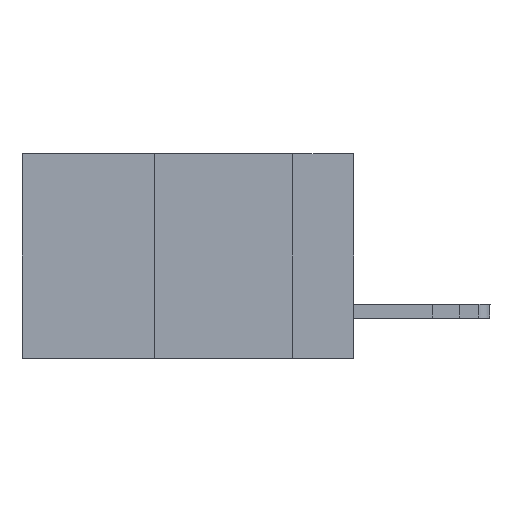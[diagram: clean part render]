
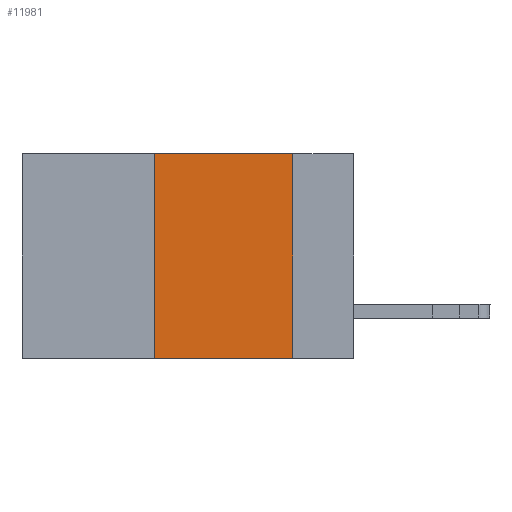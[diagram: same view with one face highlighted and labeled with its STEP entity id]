
A CAD part, left-side view. The second image highlights one B-rep face of the part: STEP entity #11981.
In plain terms, the highlighted planar face has unit normal (-1, 0, 0).
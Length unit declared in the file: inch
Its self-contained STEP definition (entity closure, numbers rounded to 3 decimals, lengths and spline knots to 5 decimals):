
#459 = ORIENTED_EDGE ( 'NONE', *, *, #1982, .F. ) ;
#484 = ORIENTED_EDGE ( 'NONE', *, *, #7917, .F. ) ;
#525 = CARTESIAN_POINT ( 'NONE',  ( 0., 0.6, 0. ) ) ;
#664 = ORIENTED_EDGE ( 'NONE', *, *, #16163, .T. ) ;
#945 = CARTESIAN_POINT ( 'NONE',  ( 0., 0.36, 0. ) ) ;
#1166 = CARTESIAN_POINT ( 'NONE',  ( 0., 0.11, 0. ) ) ;
#1393 = VERTEX_POINT ( 'NONE', #12732 ) ;
#1544 = EDGE_LOOP ( 'NONE', ( #459, #9852, #484, #664 ) ) ;
#1982 = EDGE_CURVE ( 'NONE', #1393, #10221, #14683, .T. ) ;
#2704 = VERTEX_POINT ( 'NONE', #945 ) ;
#2792 = PLANE ( 'NONE',  #5031 ) ;
#3411 = CARTESIAN_POINT ( 'NONE',  ( 0., 0.6, -0.37 ) ) ;
#4093 = DIRECTION ( 'NONE',  ( 0., 0., -1. ) ) ;
#4200 = DIRECTION ( 'NONE',  ( 1., 0., 0. ) ) ;
#4222 = DIRECTION ( 'NONE',  ( 0., -1., 0. ) ) ;
#5031 = AXIS2_PLACEMENT_3D ( 'NONE', #11901, #4200, #4093 ) ;
#5520 = CARTESIAN_POINT ( 'NONE',  ( 0., 0.11, -0.37 ) ) ;
#6100 = VECTOR ( 'NONE', #12401, 39.37008 ) ;
#6307 = DIRECTION ( 'NONE',  ( 0., 0., -1. ) ) ;
#7917 = EDGE_CURVE ( 'NONE', #14417, #2704, #11323, .T. ) ;
#9029 = VECTOR ( 'NONE', #6307, 39.37008 ) ;
#9341 = DIRECTION ( 'NONE',  ( 0., 0., 1. ) ) ;
#9852 = ORIENTED_EDGE ( 'NONE', *, *, #11489, .F. ) ;
#10125 = CARTESIAN_POINT ( 'NONE',  ( 0., 0.36, -0.37 ) ) ;
#10221 = VERTEX_POINT ( 'NONE', #5520 ) ;
#10917 = VECTOR ( 'NONE', #4222, 39.37008 ) ;
#11323 = LINE ( 'NONE', #15772, #14731 ) ;
#11489 = EDGE_CURVE ( 'NONE', #2704, #1393, #14545, .T. ) ;
#11901 = CARTESIAN_POINT ( 'NONE',  ( 0., 0.6, 0. ) ) ;
#11981 = ADVANCED_FACE ( 'NONE', ( #13102 ), #2792, .F. ) ;
#12401 = DIRECTION ( 'NONE',  ( 0., -1., 0. ) ) ;
#12582 = LINE ( 'NONE', #3411, #6100 ) ;
#12732 = CARTESIAN_POINT ( 'NONE',  ( 0., 0.11, 0. ) ) ;
#13102 = FACE_OUTER_BOUND ( 'NONE', #1544, .T. ) ;
#14417 = VERTEX_POINT ( 'NONE', #10125 ) ;
#14545 = LINE ( 'NONE', #525, #10917 ) ;
#14683 = LINE ( 'NONE', #1166, #9029 ) ;
#14731 = VECTOR ( 'NONE', #9341, 39.37008 ) ;
#15772 = CARTESIAN_POINT ( 'NONE',  ( 0., 0.36, 0. ) ) ;
#16163 = EDGE_CURVE ( 'NONE', #14417, #10221, #12582, .T. ) ;
